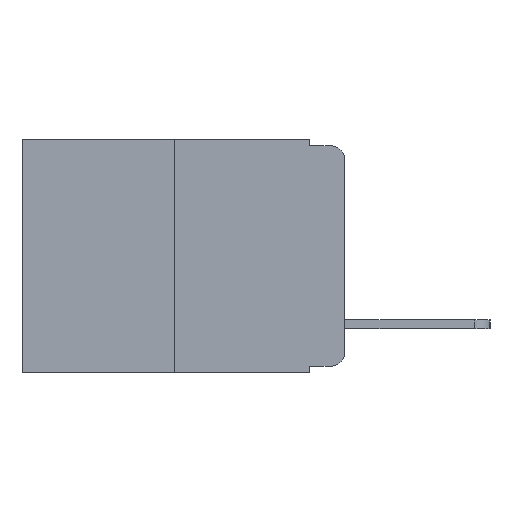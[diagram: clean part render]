
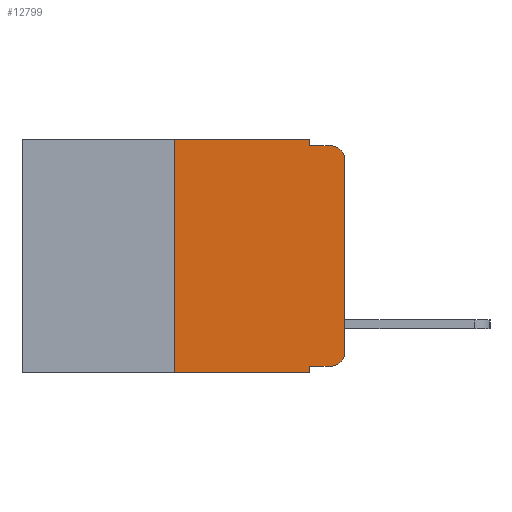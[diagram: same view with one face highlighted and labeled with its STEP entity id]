
A CAD part, left-side view. The second image highlights one B-rep face of the part: STEP entity #12799.
In plain terms, the highlighted planar face has unit normal (-1, 0, 0).
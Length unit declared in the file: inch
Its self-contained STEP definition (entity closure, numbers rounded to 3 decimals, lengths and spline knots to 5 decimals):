
#123 = AXIS2_PLACEMENT_3D ( 'NONE', #14720, #5355, #16238 ) ;
#569 = CARTESIAN_POINT ( 'NONE',  ( 0., 0.051, -0.01 ) ) ;
#693 = DIRECTION ( 'NONE',  ( 0., -1., 0. ) ) ;
#740 = CARTESIAN_POINT ( 'NONE',  ( 0., 0.02, -0.333 ) ) ;
#1204 = DIRECTION ( 'NONE',  ( 0., 0., -1. ) ) ;
#1226 = DIRECTION ( 'NONE',  ( -1., 0., 0. ) ) ;
#1424 = EDGE_CURVE ( 'NONE', #10879, #11820, #16663, .T. ) ;
#1651 = CARTESIAN_POINT ( 'NONE',  ( 0., 0.02, -0.03 ) ) ;
#1833 = VERTEX_POINT ( 'NONE', #740 ) ;
#1928 = EDGE_CURVE ( 'NONE', #9010, #5696, #14260, .T. ) ;
#2120 = DIRECTION ( 'NONE',  ( 0., -1., 0. ) ) ;
#2373 = FACE_OUTER_BOUND ( 'NONE', #12876, .T. ) ;
#2374 = CARTESIAN_POINT ( 'NONE',  ( 0., 0.051, -0.343 ) ) ;
#2821 = CARTESIAN_POINT ( 'NONE',  ( 0., 0.25, 0. ) ) ;
#2826 = VECTOR ( 'NONE', #19372, 39.37008 ) ;
#3129 = CARTESIAN_POINT ( 'NONE',  ( 0., 0.25, -0.343 ) ) ;
#3143 = ORIENTED_EDGE ( 'NONE', *, *, #19578, .F. ) ;
#3145 = CARTESIAN_POINT ( 'NONE',  ( 0., 0.051, 0. ) ) ;
#3279 = VECTOR ( 'NONE', #693, 39.37008 ) ;
#3414 = DIRECTION ( 'NONE',  ( 0., -1., 0. ) ) ;
#3705 = ORIENTED_EDGE ( 'NONE', *, *, #7109, .F. ) ;
#4419 = DIRECTION ( 'NONE',  ( 0., 0., 1. ) ) ;
#4550 = ORIENTED_EDGE ( 'NONE', *, *, #18476, .T. ) ;
#4729 = CARTESIAN_POINT ( 'NONE',  ( 0., 0.051, 0. ) ) ;
#4861 = CARTESIAN_POINT ( 'NONE',  ( 0., 0.051, 0. ) ) ;
#5315 = ORIENTED_EDGE ( 'NONE', *, *, #9233, .T. ) ;
#5355 = DIRECTION ( 'NONE',  ( -1., 0., 0. ) ) ;
#5696 = VERTEX_POINT ( 'NONE', #15727 ) ;
#6224 = PLANE ( 'NONE',  #19521 ) ;
#6277 = VECTOR ( 'NONE', #4419, 39.37008 ) ;
#6518 = DIRECTION ( 'NONE',  ( 0., 0., -1. ) ) ;
#6943 = AXIS2_PLACEMENT_3D ( 'NONE', #1651, #1226, #1204 ) ;
#7109 = EDGE_CURVE ( 'NONE', #15934, #8164, #12638, .T. ) ;
#7185 = LINE ( 'NONE', #3145, #14481 ) ;
#7477 = VECTOR ( 'NONE', #3414, 39.37008 ) ;
#7712 = EDGE_CURVE ( 'NONE', #1833, #16175, #13330, .T. ) ;
#7812 = DIRECTION ( 'NONE',  ( 1., 0., 0. ) ) ;
#7834 = DIRECTION ( 'NONE',  ( 0., 0., 1. ) ) ;
#8164 = VERTEX_POINT ( 'NONE', #4861 ) ;
#8468 = VECTOR ( 'NONE', #16203, 39.37008 ) ;
#9010 = VERTEX_POINT ( 'NONE', #19583 ) ;
#9233 = EDGE_CURVE ( 'NONE', #16175, #9010, #12542, .T. ) ;
#9283 = CARTESIAN_POINT ( 'NONE',  ( 0., 0.473, 0. ) ) ;
#10877 = LINE ( 'NONE', #569, #18978 ) ;
#10879 = VERTEX_POINT ( 'NONE', #13667 ) ;
#10947 = CARTESIAN_POINT ( 'NONE',  ( 0., 0., 0. ) ) ;
#11696 = CARTESIAN_POINT ( 'NONE',  ( 0., 0.473, 0. ) ) ;
#11820 = VERTEX_POINT ( 'NONE', #2374 ) ;
#12131 = ORIENTED_EDGE ( 'NONE', *, *, #1424, .F. ) ;
#12523 = ORIENTED_EDGE ( 'NONE', *, *, #14223, .T. ) ;
#12542 = LINE ( 'NONE', #10947, #13020 ) ;
#12638 = LINE ( 'NONE', #11696, #3279 ) ;
#12723 = ORIENTED_EDGE ( 'NONE', *, *, #1928, .T. ) ;
#12799 = ADVANCED_FACE ( 'NONE', ( #2373 ), #6224, .F. ) ;
#12846 = CARTESIAN_POINT ( 'NONE',  ( 0., 0.473, -0.343 ) ) ;
#12876 = EDGE_LOOP ( 'NONE', ( #5315, #12723, #3143, #18651, #3705, #13128, #12523, #12131, #4550, #14797 ) ) ;
#13020 = VECTOR ( 'NONE', #7834, 39.37008 ) ;
#13128 = ORIENTED_EDGE ( 'NONE', *, *, #13907, .F. ) ;
#13245 = CARTESIAN_POINT ( 'NONE',  ( 0., 0., -0.313 ) ) ;
#13330 = CIRCLE ( 'NONE', #123, 0.02 ) ;
#13667 = CARTESIAN_POINT ( 'NONE',  ( 0., 0.051, -0.333 ) ) ;
#13907 = EDGE_CURVE ( 'NONE', #18755, #15934, #15026, .T. ) ;
#14223 = EDGE_CURVE ( 'NONE', #18755, #11820, #19213, .T. ) ;
#14260 = CIRCLE ( 'NONE', #6943, 0.02 ) ;
#14481 = VECTOR ( 'NONE', #6518, 39.37008 ) ;
#14720 = CARTESIAN_POINT ( 'NONE',  ( 0., 0.02, -0.313 ) ) ;
#14797 = ORIENTED_EDGE ( 'NONE', *, *, #7712, .T. ) ;
#14851 = LINE ( 'NONE', #14873, #2826 ) ;
#14873 = CARTESIAN_POINT ( 'NONE',  ( 0., 0.051, -0.333 ) ) ;
#15026 = LINE ( 'NONE', #2821, #6277 ) ;
#15727 = CARTESIAN_POINT ( 'NONE',  ( 0., 0.02, -0.01 ) ) ;
#15736 = CARTESIAN_POINT ( 'NONE',  ( 0., 0.25, 0. ) ) ;
#15934 = VERTEX_POINT ( 'NONE', #15736 ) ;
#15959 = EDGE_CURVE ( 'NONE', #8164, #19860, #7185, .T. ) ;
#16175 = VERTEX_POINT ( 'NONE', #13245 ) ;
#16203 = DIRECTION ( 'NONE',  ( 0., 0., -1. ) ) ;
#16238 = DIRECTION ( 'NONE',  ( 0., 0., -1. ) ) ;
#16663 = LINE ( 'NONE', #4729, #8468 ) ;
#16940 = CARTESIAN_POINT ( 'NONE',  ( 0., 0.051, -0.01 ) ) ;
#18476 = EDGE_CURVE ( 'NONE', #10879, #1833, #14851, .T. ) ;
#18529 = DIRECTION ( 'NONE',  ( 0., 0., -1. ) ) ;
#18651 = ORIENTED_EDGE ( 'NONE', *, *, #15959, .F. ) ;
#18755 = VERTEX_POINT ( 'NONE', #3129 ) ;
#18978 = VECTOR ( 'NONE', #2120, 39.37008 ) ;
#19213 = LINE ( 'NONE', #12846, #7477 ) ;
#19372 = DIRECTION ( 'NONE',  ( 0., -1., 0. ) ) ;
#19521 = AXIS2_PLACEMENT_3D ( 'NONE', #9283, #7812, #18529 ) ;
#19578 = EDGE_CURVE ( 'NONE', #19860, #5696, #10877, .T. ) ;
#19583 = CARTESIAN_POINT ( 'NONE',  ( 0., 0., -0.03 ) ) ;
#19860 = VERTEX_POINT ( 'NONE', #16940 ) ;
